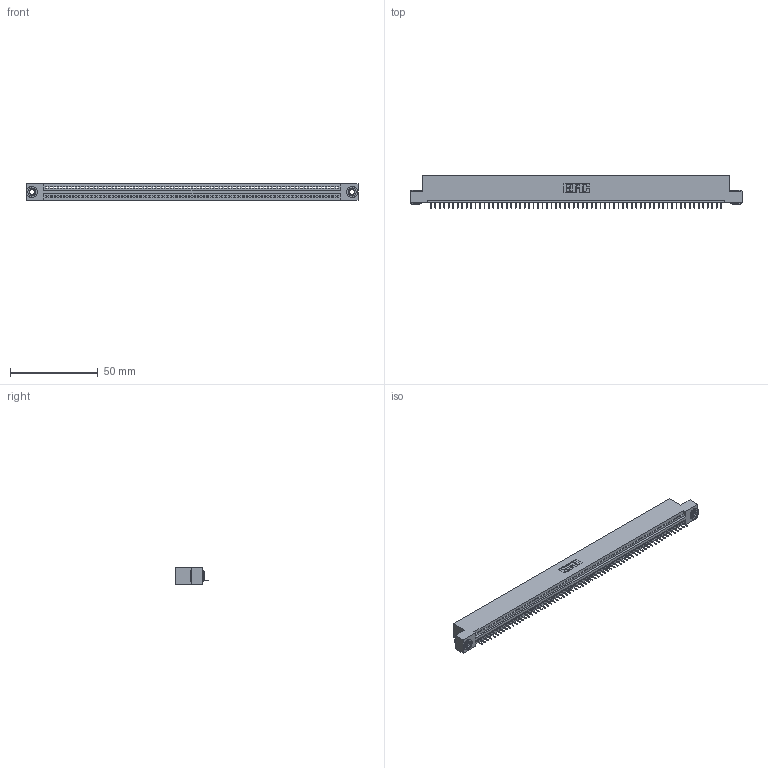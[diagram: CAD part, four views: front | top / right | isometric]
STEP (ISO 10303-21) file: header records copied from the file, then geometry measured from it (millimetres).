
FILE_DESCRIPTION (( 'STEP AP203' ), '1' );
FILE_NAME ('895-066-525-103.STEP', '2020-09-28T12:55:34', ( '' ), ( '' ), 'SwSTEP 2.0', 'SolidWorks 2020', '' );
FILE_SCHEMA (( 'CONFIG_CONTROL_DESIGN' ));
Length unit declared in the file: inch
Products named in the file (4): 895-066-525-103; 845 Part_Flush Mounting Lugs - 0.156 Dia-TH; 345-250-002_345-250-002-102; 345-292-001_345-293-125
Assembly tree (69 placements, depth 2):
  895-066-525-103
    845 Part_Flush Mounting Lugs - 0.156 Dia-TH
    345-292-001_345-293-125  x66
    345-250-002_345-250-002-102  x2
Bounding box: 188.85 x 18.72 x 9.4 mm (x, y, z)
Volume: 17883.6 mm3; surface area: 23407.7 mm2
Topology: 69 solids, 69 shells, 4256 faces, 12297 edges, 7930 vertices
Faces by surface type: plane 3126, cylinder 1122, cone 8
Entity records: 47166 total; most frequent: CARTESIAN_POINT 8145, ORIENTED_EDGE 8138, DIRECTION 7111, EDGE_CURVE 4069, LINE 3653, VECTOR 3653, VERTEX_POINT 2706, AXIS2_PLACEMENT_3D 1729
